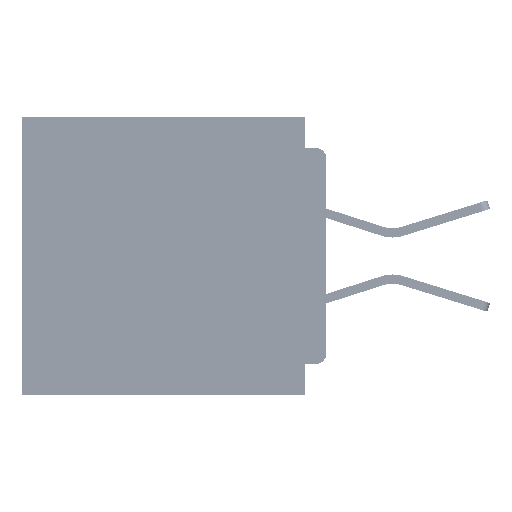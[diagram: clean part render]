
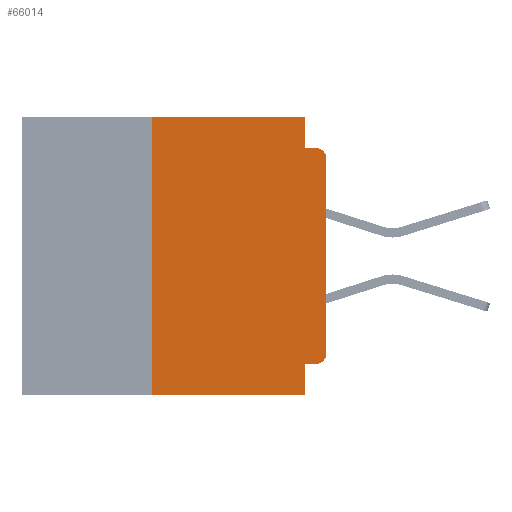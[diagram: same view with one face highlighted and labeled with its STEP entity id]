
A CAD part, left-side view. The second image highlights one B-rep face of the part: STEP entity #66014.
In plain terms, the highlighted planar face has unit normal (-1, 0, 0).
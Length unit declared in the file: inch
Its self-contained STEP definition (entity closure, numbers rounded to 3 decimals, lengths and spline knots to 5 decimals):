
#3098 = LINE ( 'NONE', #35168, #39301 ) ;
#4019 = CARTESIAN_POINT ( 'NONE',  ( 0., 0., -0.355 ) ) ;
#5477 = ORIENTED_EDGE ( 'NONE', *, *, #51197, .F. ) ;
#6253 = VERTEX_POINT ( 'NONE', #36364 ) ;
#6293 = CARTESIAN_POINT ( 'NONE',  ( 0., 0.25, 0. ) ) ;
#8930 = CARTESIAN_POINT ( 'NONE',  ( 0., 0.031, -0.355 ) ) ;
#9421 = CARTESIAN_POINT ( 'NONE',  ( 0., 0.015, -0.34 ) ) ;
#9729 = VERTEX_POINT ( 'NONE', #44352 ) ;
#9771 = PLANE ( 'NONE',  #27573 ) ;
#10755 = EDGE_CURVE ( 'NONE', #6253, #18369, #53160, .T. ) ;
#11278 = VERTEX_POINT ( 'NONE', #8930 ) ;
#12498 = EDGE_CURVE ( 'NONE', #21452, #9729, #15455, .T. ) ;
#12613 = ORIENTED_EDGE ( 'NONE', *, *, #23572, .F. ) ;
#12902 = VECTOR ( 'NONE', #64131, 39.37008 ) ;
#13218 = CARTESIAN_POINT ( 'NONE',  ( 0., 0.031, -0.4 ) ) ;
#13960 = DIRECTION ( 'NONE',  ( -1., 0., 0. ) ) ;
#14622 = DIRECTION ( 'NONE',  ( 0., 0., -1. ) ) ;
#14971 = CARTESIAN_POINT ( 'NONE',  ( 0., 0.437, 0. ) ) ;
#15455 = CIRCLE ( 'NONE', #22846, 0.015 ) ;
#15504 = ORIENTED_EDGE ( 'NONE', *, *, #12498, .T. ) ;
#16192 = DIRECTION ( 'NONE',  ( 0., -1., 0. ) ) ;
#16221 = FACE_OUTER_BOUND ( 'NONE', #54333, .T. ) ;
#16773 = LINE ( 'NONE', #64709, #28769 ) ;
#16918 = CARTESIAN_POINT ( 'NONE',  ( 0., 0.437, 0. ) ) ;
#17418 = EDGE_CURVE ( 'NONE', #6253, #11278, #65961, .T. ) ;
#17929 = LINE ( 'NONE', #46750, #55355 ) ;
#18279 = CARTESIAN_POINT ( 'NONE',  ( 0., 0.031, -0.045 ) ) ;
#18369 = VERTEX_POINT ( 'NONE', #48009 ) ;
#20131 = DIRECTION ( 'NONE',  ( 0., 0., -1. ) ) ;
#20655 = EDGE_CURVE ( 'NONE', #55604, #42565, #17929, .T. ) ;
#21452 = VERTEX_POINT ( 'NONE', #37785 ) ;
#22105 = VERTEX_POINT ( 'NONE', #29604 ) ;
#22128 = VECTOR ( 'NONE', #50479, 39.37008 ) ;
#22846 = AXIS2_PLACEMENT_3D ( 'NONE', #44561, #13960, #49642 ) ;
#23572 = EDGE_CURVE ( 'NONE', #47319, #22105, #39255, .T. ) ;
#23730 = LINE ( 'NONE', #45620, #22128 ) ;
#25670 = VECTOR ( 'NONE', #52534, 39.37008 ) ;
#25899 = EDGE_CURVE ( 'NONE', #62904, #9729, #23730, .T. ) ;
#26566 = LINE ( 'NONE', #28681, #12902 ) ;
#27573 = AXIS2_PLACEMENT_3D ( 'NONE', #14971, #50615, #20131 ) ;
#27695 = ORIENTED_EDGE ( 'NONE', *, *, #17418, .F. ) ;
#28681 = CARTESIAN_POINT ( 'NONE',  ( 0., 0.031, 0. ) ) ;
#28769 = VECTOR ( 'NONE', #29265, 39.37008 ) ;
#29265 = DIRECTION ( 'NONE',  ( 0., 0., 1. ) ) ;
#29604 = CARTESIAN_POINT ( 'NONE',  ( 0., 0.031, 0. ) ) ;
#31746 = EDGE_CURVE ( 'NONE', #18369, #21452, #16773, .T. ) ;
#35168 = CARTESIAN_POINT ( 'NONE',  ( 0., 0.25, -0.4 ) ) ;
#36364 = CARTESIAN_POINT ( 'NONE',  ( 0., 0.015, -0.355 ) ) ;
#37351 = AXIS2_PLACEMENT_3D ( 'NONE', #9421, #45214, #14622 ) ;
#37785 = CARTESIAN_POINT ( 'NONE',  ( 0., 0., -0.06 ) ) ;
#39255 = LINE ( 'NONE', #16918, #25670 ) ;
#39301 = VECTOR ( 'NONE', #50444, 39.37008 ) ;
#41472 = EDGE_CURVE ( 'NONE', #11278, #42565, #55744, .T. ) ;
#42310 = VECTOR ( 'NONE', #59098, 39.37008 ) ;
#42565 = VERTEX_POINT ( 'NONE', #63751 ) ;
#43343 = ORIENTED_EDGE ( 'NONE', *, *, #41472, .F. ) ;
#44352 = CARTESIAN_POINT ( 'NONE',  ( 0., 0.015, -0.045 ) ) ;
#44561 = CARTESIAN_POINT ( 'NONE',  ( 0., 0.015, -0.06 ) ) ;
#45214 = DIRECTION ( 'NONE',  ( -1., 0., 0. ) ) ;
#45620 = CARTESIAN_POINT ( 'NONE',  ( 0., 0., -0.045 ) ) ;
#46750 = CARTESIAN_POINT ( 'NONE',  ( 0., 0.437, -0.4 ) ) ;
#47319 = VERTEX_POINT ( 'NONE', #6293 ) ;
#48009 = CARTESIAN_POINT ( 'NONE',  ( 0., 0., -0.34 ) ) ;
#48734 = ORIENTED_EDGE ( 'NONE', *, *, #51402, .F. ) ;
#49642 = DIRECTION ( 'NONE',  ( 0., 0., -1. ) ) ;
#49888 = ORIENTED_EDGE ( 'NONE', *, *, #31746, .T. ) ;
#50393 = ORIENTED_EDGE ( 'NONE', *, *, #20655, .T. ) ;
#50444 = DIRECTION ( 'NONE',  ( 0., 0., 1. ) ) ;
#50479 = DIRECTION ( 'NONE',  ( 0., -1., 0. ) ) ;
#50615 = DIRECTION ( 'NONE',  ( 1., 0., 0. ) ) ;
#51197 = EDGE_CURVE ( 'NONE', #22105, #62904, #26566, .T. ) ;
#51402 = EDGE_CURVE ( 'NONE', #55604, #47319, #3098, .T. ) ;
#52534 = DIRECTION ( 'NONE',  ( 0., -1., 0. ) ) ;
#52544 = VECTOR ( 'NONE', #55214, 39.37008 ) ;
#53160 = CIRCLE ( 'NONE', #37351, 0.015 ) ;
#54153 = ORIENTED_EDGE ( 'NONE', *, *, #10755, .T. ) ;
#54333 = EDGE_LOOP ( 'NONE', ( #49888, #15504, #62427, #5477, #12613, #48734, #50393, #43343, #27695, #54153 ) ) ;
#55214 = DIRECTION ( 'NONE',  ( 0., 1., 0. ) ) ;
#55355 = VECTOR ( 'NONE', #16192, 39.37008 ) ;
#55604 = VERTEX_POINT ( 'NONE', #64935 ) ;
#55744 = LINE ( 'NONE', #13218, #42310 ) ;
#59098 = DIRECTION ( 'NONE',  ( 0., 0., -1. ) ) ;
#62427 = ORIENTED_EDGE ( 'NONE', *, *, #25899, .F. ) ;
#62904 = VERTEX_POINT ( 'NONE', #18279 ) ;
#63751 = CARTESIAN_POINT ( 'NONE',  ( 0., 0.031, -0.4 ) ) ;
#64131 = DIRECTION ( 'NONE',  ( 0., 0., -1. ) ) ;
#64709 = CARTESIAN_POINT ( 'NONE',  ( 0., 0., 0. ) ) ;
#64935 = CARTESIAN_POINT ( 'NONE',  ( 0., 0.25, -0.4 ) ) ;
#65961 = LINE ( 'NONE', #4019, #52544 ) ;
#66014 = ADVANCED_FACE ( 'NONE', ( #16221 ), #9771, .F. ) ;
